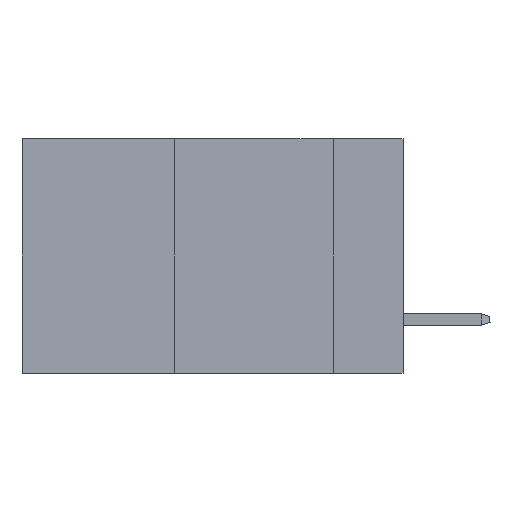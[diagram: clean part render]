
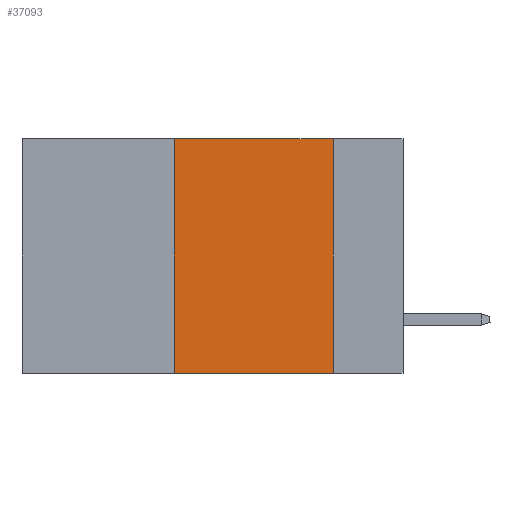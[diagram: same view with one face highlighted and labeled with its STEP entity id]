
A CAD part, left-side view. The second image highlights one B-rep face of the part: STEP entity #37093.
In plain terms, the highlighted planar face has unit normal (-1, 0, 0).
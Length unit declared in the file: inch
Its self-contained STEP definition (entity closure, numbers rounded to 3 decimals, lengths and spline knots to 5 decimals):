
#486 = CARTESIAN_POINT ( 'NONE',  ( 0., 0.11, 0. ) ) ;
#1452 = ORIENTED_EDGE ( 'NONE', *, *, #30807, .T. ) ;
#2380 = LINE ( 'NONE', #21530, #46807 ) ;
#2771 = CARTESIAN_POINT ( 'NONE',  ( 0., 0.11, 0. ) ) ;
#3750 = EDGE_LOOP ( 'NONE', ( #37166, #27528, #35322, #1452 ) ) ;
#5357 = CARTESIAN_POINT ( 'NONE',  ( 0., 0.6, 0. ) ) ;
#6957 = VECTOR ( 'NONE', #15453, 39.37008 ) ;
#8124 = DIRECTION ( 'NONE',  ( 0., 0., 1. ) ) ;
#8229 = VECTOR ( 'NONE', #18448, 39.37008 ) ;
#8255 = VERTEX_POINT ( 'NONE', #19578 ) ;
#8527 = CARTESIAN_POINT ( 'NONE',  ( 0., 0.36, -0.37 ) ) ;
#13439 = VERTEX_POINT ( 'NONE', #2771 ) ;
#14996 = CARTESIAN_POINT ( 'NONE',  ( 0., 0.36, 0. ) ) ;
#15453 = DIRECTION ( 'NONE',  ( 0., 0., -1. ) ) ;
#16411 = DIRECTION ( 'NONE',  ( 0., 0., -1. ) ) ;
#16650 = EDGE_CURVE ( 'NONE', #13439, #44418, #22838, .T. ) ;
#18448 = DIRECTION ( 'NONE',  ( 0., -1., 0. ) ) ;
#18561 = DIRECTION ( 'NONE',  ( 0., -1., 0. ) ) ;
#19578 = CARTESIAN_POINT ( 'NONE',  ( 0., 0.36, 0. ) ) ;
#20097 = PLANE ( 'NONE',  #25016 ) ;
#21530 = CARTESIAN_POINT ( 'NONE',  ( 0., 0.6, 0. ) ) ;
#22376 = LINE ( 'NONE', #48139, #8229 ) ;
#22838 = LINE ( 'NONE', #486, #6957 ) ;
#25016 = AXIS2_PLACEMENT_3D ( 'NONE', #5357, #46570, #16411 ) ;
#25674 = EDGE_CURVE ( 'NONE', #29105, #8255, #41003, .T. ) ;
#27528 = ORIENTED_EDGE ( 'NONE', *, *, #35492, .F. ) ;
#29105 = VERTEX_POINT ( 'NONE', #8527 ) ;
#30807 = EDGE_CURVE ( 'NONE', #29105, #44418, #22376, .T. ) ;
#35322 = ORIENTED_EDGE ( 'NONE', *, *, #25674, .F. ) ;
#35492 = EDGE_CURVE ( 'NONE', #8255, #13439, #2380, .T. ) ;
#36064 = CARTESIAN_POINT ( 'NONE',  ( 0., 0.11, -0.37 ) ) ;
#37093 = ADVANCED_FACE ( 'NONE', ( #42885 ), #20097, .F. ) ;
#37166 = ORIENTED_EDGE ( 'NONE', *, *, #16650, .F. ) ;
#41003 = LINE ( 'NONE', #14996, #44901 ) ;
#42885 = FACE_OUTER_BOUND ( 'NONE', #3750, .T. ) ;
#44418 = VERTEX_POINT ( 'NONE', #36064 ) ;
#44901 = VECTOR ( 'NONE', #8124, 39.37008 ) ;
#46570 = DIRECTION ( 'NONE',  ( 1., 0., 0. ) ) ;
#46807 = VECTOR ( 'NONE', #18561, 39.37008 ) ;
#48139 = CARTESIAN_POINT ( 'NONE',  ( 0., 0.6, -0.37 ) ) ;
